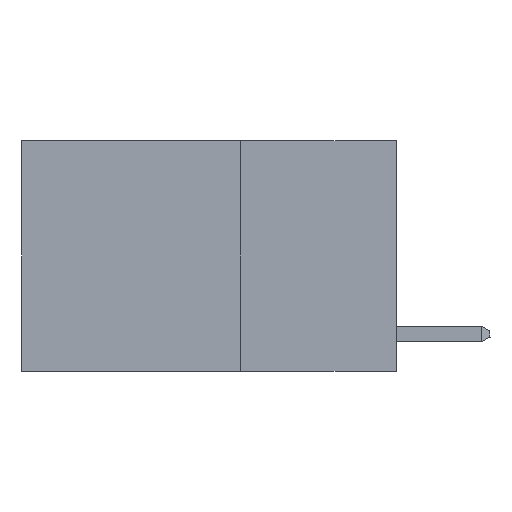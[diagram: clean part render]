
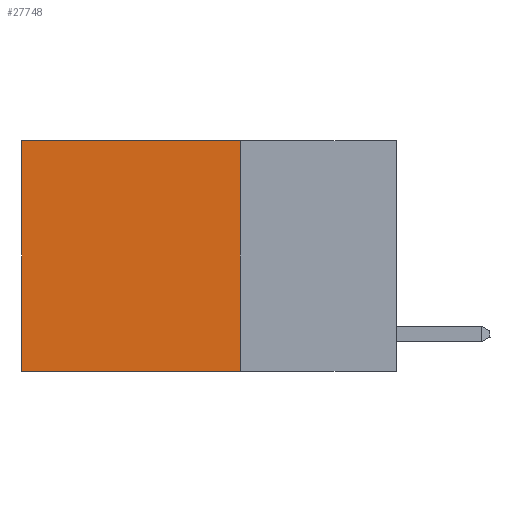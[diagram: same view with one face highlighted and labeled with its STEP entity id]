
A CAD part, left-side view. The second image highlights one B-rep face of the part: STEP entity #27748.
In plain terms, the highlighted planar face has unit normal (-1, 0, 0).
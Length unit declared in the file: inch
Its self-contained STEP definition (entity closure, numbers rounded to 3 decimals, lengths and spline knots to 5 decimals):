
#127 = ORIENTED_EDGE ( 'NONE', *, *, #13342, .T. ) ;
#275 = LINE ( 'NONE', #17543, #12338 ) ;
#665 = EDGE_CURVE ( 'NONE', #21637, #13271, #28349, .T. ) ;
#1893 = VERTEX_POINT ( 'NONE', #3763 ) ;
#3323 = CARTESIAN_POINT ( 'NONE',  ( 0.2625, 0.25, 0. ) ) ;
#3763 = CARTESIAN_POINT ( 'NONE',  ( 0.2625, 0.6, 0. ) ) ;
#3793 = VERTEX_POINT ( 'NONE', #26513 ) ;
#4457 = VECTOR ( 'NONE', #20262, 39.37008 ) ;
#5687 = ORIENTED_EDGE ( 'NONE', *, *, #18693, .F. ) ;
#7369 = EDGE_CURVE ( 'NONE', #1893, #3793, #28863, .T. ) ;
#7437 = ORIENTED_EDGE ( 'NONE', *, *, #665, .F. ) ;
#7473 = AXIS2_PLACEMENT_3D ( 'NONE', #27734, #13682, #30017 ) ;
#8314 = CARTESIAN_POINT ( 'NONE',  ( 0.2625, 0.6, 0. ) ) ;
#8859 = PLANE ( 'NONE',  #7473 ) ;
#8887 = DIRECTION ( 'NONE',  ( 0., 0., -1. ) ) ;
#11555 = VECTOR ( 'NONE', #18065, 39.37008 ) ;
#12338 = VECTOR ( 'NONE', #19966, 39.37008 ) ;
#12769 = ORIENTED_EDGE ( 'NONE', *, *, #7369, .T. ) ;
#13271 = VERTEX_POINT ( 'NONE', #27103 ) ;
#13342 = EDGE_CURVE ( 'NONE', #21637, #1893, #24147, .T. ) ;
#13682 = DIRECTION ( 'NONE',  ( 1., 0., 0. ) ) ;
#15668 = CARTESIAN_POINT ( 'NONE',  ( 0.2625, 0.25, 0. ) ) ;
#15751 = FACE_OUTER_BOUND ( 'NONE', #23264, .T. ) ;
#17543 = CARTESIAN_POINT ( 'NONE',  ( 0.2625, 0.25, -0.37 ) ) ;
#18065 = DIRECTION ( 'NONE',  ( 0., 1., 0. ) ) ;
#18521 = CARTESIAN_POINT ( 'NONE',  ( 0.2625, 0.25, 0. ) ) ;
#18693 = EDGE_CURVE ( 'NONE', #13271, #3793, #275, .T. ) ;
#19966 = DIRECTION ( 'NONE',  ( 0., 1., 0. ) ) ;
#20262 = DIRECTION ( 'NONE',  ( 0., 0., -1. ) ) ;
#21637 = VERTEX_POINT ( 'NONE', #3323 ) ;
#23264 = EDGE_LOOP ( 'NONE', ( #12769, #5687, #7437, #127 ) ) ;
#24147 = LINE ( 'NONE', #15668, #11555 ) ;
#26513 = CARTESIAN_POINT ( 'NONE',  ( 0.2625, 0.6, -0.37 ) ) ;
#27103 = CARTESIAN_POINT ( 'NONE',  ( 0.2625, 0.25, -0.37 ) ) ;
#27734 = CARTESIAN_POINT ( 'NONE',  ( 0.2625, 0.25, 0. ) ) ;
#27748 = ADVANCED_FACE ( 'NONE', ( #15751 ), #8859, .F. ) ;
#28349 = LINE ( 'NONE', #18521, #30489 ) ;
#28863 = LINE ( 'NONE', #8314, #4457 ) ;
#30017 = DIRECTION ( 'NONE',  ( 0., 0., -1. ) ) ;
#30489 = VECTOR ( 'NONE', #8887, 39.37008 ) ;
